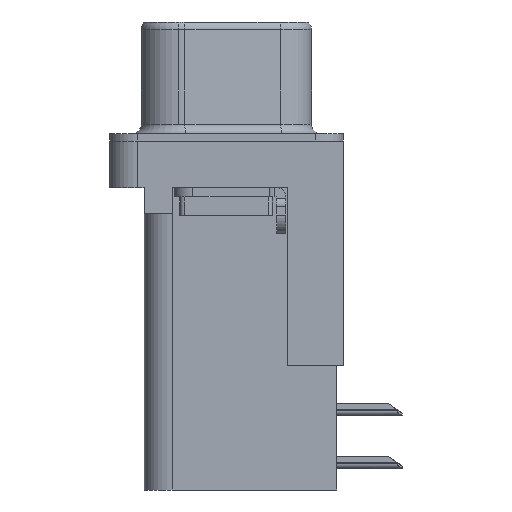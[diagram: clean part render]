
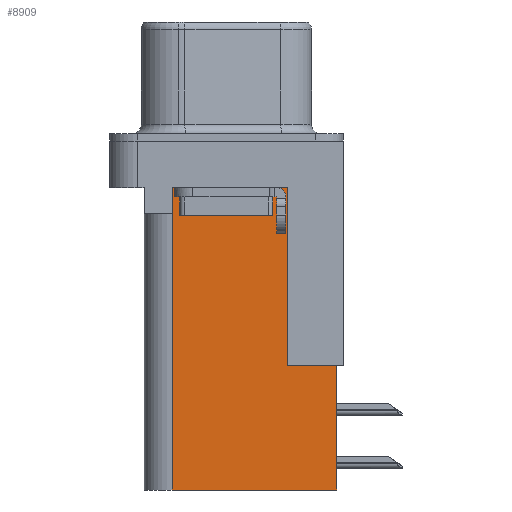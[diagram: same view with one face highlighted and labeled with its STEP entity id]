
A CAD part, left-side view. The second image highlights one B-rep face of the part: STEP entity #8909.
In plain terms, the highlighted planar face has unit normal (-1, 0, 0).
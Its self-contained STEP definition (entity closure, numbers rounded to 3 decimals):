
#623 = ORIENTED_EDGE ( 'NONE', *, *, #7248, .T. ) ;
#825 = VECTOR ( 'NONE', #21378, 1000. ) ;
#847 = LINE ( 'NONE', #16191, #825 ) ;
#938 = VECTOR ( 'NONE', #19168, 1000. ) ;
#1338 = VECTOR ( 'NONE', #15833, 1000. ) ;
#1368 = LINE ( 'NONE', #19185, #1338 ) ;
#1546 = VECTOR ( 'NONE', #15168, 1000. ) ;
#3020 = VERTEX_POINT ( 'NONE', #5250 ) ;
#3134 = CARTESIAN_POINT ( 'NONE',  ( 3.7, -3.295, -2.5 ) ) ;
#3187 = FACE_OUTER_BOUND ( 'NONE', #16211, .T. ) ;
#3347 = EDGE_CURVE ( 'NONE', #20774, #3960, #5789, .T. ) ;
#3399 = ORIENTED_EDGE ( 'NONE', *, *, #22119, .T. ) ;
#3722 = CARTESIAN_POINT ( 'NONE',  ( 3.7, 2.895, -3.9 ) ) ;
#3847 = CARTESIAN_POINT ( 'NONE',  ( 3.7, 2.895, -3.9 ) ) ;
#3960 = VERTEX_POINT ( 'NONE', #14875 ) ;
#4549 = DIRECTION ( 'NONE',  ( 0., 0., -1. ) ) ;
#4845 = EDGE_CURVE ( 'NONE', #12370, #13246, #19943, .T. ) ;
#4886 = VECTOR ( 'NONE', #22334, 1000. ) ;
#5098 = CARTESIAN_POINT ( 'NONE',  ( 3.7, -6.295, -12.05 ) ) ;
#5250 = CARTESIAN_POINT ( 'NONE',  ( 3.7, -3.295, -2.5 ) ) ;
#5439 = LINE ( 'NONE', #20528, #4886 ) ;
#5607 = CARTESIAN_POINT ( 'NONE',  ( 3.7, 2.895, -2.5 ) ) ;
#5748 = LINE ( 'NONE', #3134, #1546 ) ;
#5789 = LINE ( 'NONE', #9615, #5978 ) ;
#5880 = VERTEX_POINT ( 'NONE', #5607 ) ;
#5978 = VECTOR ( 'NONE', #10111, 1000. ) ;
#6424 = CARTESIAN_POINT ( 'NONE',  ( 3.7, -5.925, -2. ) ) ;
#7248 = EDGE_CURVE ( 'NONE', #12370, #18117, #9841, .T. ) ;
#7637 = CARTESIAN_POINT ( 'NONE',  ( 3.7, -3.295, -18.76 ) ) ;
#8909 = ADVANCED_FACE ( 'NONE', ( #3187 ), #21155, .F. ) ;
#9035 = ORIENTED_EDGE ( 'NONE', *, *, #4845, .F. ) ;
#9365 = DIRECTION ( 'NONE',  ( 0., 1., 0. ) ) ;
#9417 = EDGE_CURVE ( 'NONE', #16295, #3960, #1368, .T. ) ;
#9536 = EDGE_CURVE ( 'NONE', #18117, #3020, #847, .T. ) ;
#9615 = CARTESIAN_POINT ( 'NONE',  ( 3.7, 2.925, -18.76 ) ) ;
#9841 = LINE ( 'NONE', #5098, #9913 ) ;
#9913 = VECTOR ( 'NONE', #12002, 1000. ) ;
#10111 = DIRECTION ( 'NONE',  ( 0., 0., 1. ) ) ;
#10129 = ORIENTED_EDGE ( 'NONE', *, *, #21358, .F. ) ;
#12002 = DIRECTION ( 'NONE',  ( 0., 1., 0. ) ) ;
#12370 = VERTEX_POINT ( 'NONE', #18372 ) ;
#13246 = VERTEX_POINT ( 'NONE', #13687 ) ;
#13687 = CARTESIAN_POINT ( 'NONE',  ( 3.7, -5.925, -18.76 ) ) ;
#13928 = ORIENTED_EDGE ( 'NONE', *, *, #3347, .F. ) ;
#14875 = CARTESIAN_POINT ( 'NONE',  ( 3.7, 2.925, -3.9 ) ) ;
#15168 = DIRECTION ( 'NONE',  ( 0., 1., 0. ) ) ;
#15309 = CARTESIAN_POINT ( 'NONE',  ( 3.7, 2.925, -18.76 ) ) ;
#15833 = DIRECTION ( 'NONE',  ( 0., 1., 0. ) ) ;
#16191 = CARTESIAN_POINT ( 'NONE',  ( 3.7, -3.295, -18.76 ) ) ;
#16211 = EDGE_LOOP ( 'NONE', ( #17763, #3399, #17923, #13928, #10129, #9035, #623, #17948 ) ) ;
#16295 = VERTEX_POINT ( 'NONE', #3847 ) ;
#17763 = ORIENTED_EDGE ( 'NONE', *, *, #21087, .T. ) ;
#17923 = ORIENTED_EDGE ( 'NONE', *, *, #9417, .T. ) ;
#17948 = ORIENTED_EDGE ( 'NONE', *, *, #9536, .T. ) ;
#18117 = VERTEX_POINT ( 'NONE', #18947 ) ;
#18130 = AXIS2_PLACEMENT_3D ( 'NONE', #7637, #19488, #9365 ) ;
#18372 = CARTESIAN_POINT ( 'NONE',  ( 3.7, -5.925, -12.05 ) ) ;
#18947 = CARTESIAN_POINT ( 'NONE',  ( 3.7, -3.295, -12.05 ) ) ;
#19168 = DIRECTION ( 'NONE',  ( 0., 0., -1. ) ) ;
#19185 = CARTESIAN_POINT ( 'NONE',  ( 3.7, 0., -3.9 ) ) ;
#19488 = DIRECTION ( 'NONE',  ( 1., 0., 0. ) ) ;
#19819 = LINE ( 'NONE', #3722, #938 ) ;
#19943 = LINE ( 'NONE', #6424, #19975 ) ;
#19975 = VECTOR ( 'NONE', #4549, 1000. ) ;
#20528 = CARTESIAN_POINT ( 'NONE',  ( 3.7, -3.295, -18.76 ) ) ;
#20774 = VERTEX_POINT ( 'NONE', #15309 ) ;
#21087 = EDGE_CURVE ( 'NONE', #3020, #5880, #5748, .T. ) ;
#21155 = PLANE ( 'NONE',  #18130 ) ;
#21358 = EDGE_CURVE ( 'NONE', #13246, #20774, #5439, .T. ) ;
#21378 = DIRECTION ( 'NONE',  ( 0., 0., 1. ) ) ;
#22119 = EDGE_CURVE ( 'NONE', #5880, #16295, #19819, .T. ) ;
#22334 = DIRECTION ( 'NONE',  ( 0., 1., 0. ) ) ;
